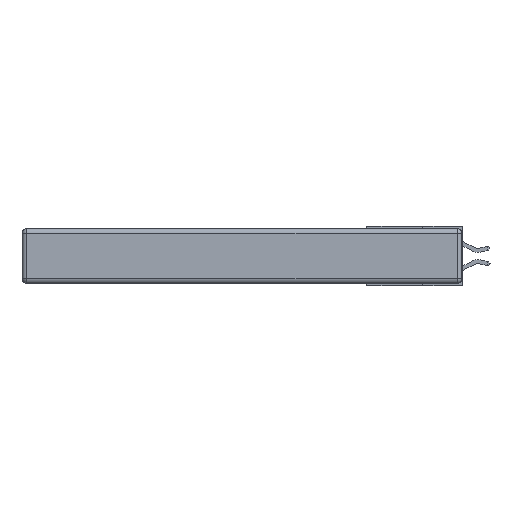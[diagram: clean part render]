
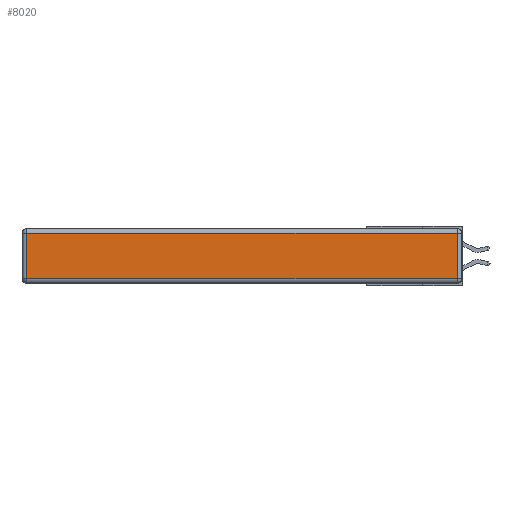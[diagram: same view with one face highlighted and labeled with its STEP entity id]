
A CAD part, left-side view. The second image highlights one B-rep face of the part: STEP entity #8020.
In plain terms, the highlighted planar face has unit normal (-1, 0, 0).
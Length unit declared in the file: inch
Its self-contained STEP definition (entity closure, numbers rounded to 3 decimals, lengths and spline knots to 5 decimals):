
#889 = LINE ( 'NONE', #14037, #1727 ) ;
#997 = CARTESIAN_POINT ( 'NONE',  ( 0., 2.72, -0.03 ) ) ;
#1402 = EDGE_CURVE ( 'NONE', #5670, #11887, #889, .T. ) ;
#1727 = VECTOR ( 'NONE', #5979, 39.37008 ) ;
#2319 = FACE_OUTER_BOUND ( 'NONE', #15746, .T. ) ;
#2559 = CARTESIAN_POINT ( 'NONE',  ( 0., 0., -0.313 ) ) ;
#3452 = DIRECTION ( 'NONE',  ( 0., 0., 1. ) ) ;
#3626 = PLANE ( 'NONE',  #10533 ) ;
#3852 = CARTESIAN_POINT ( 'NONE',  ( 0., 0.03, -0.03 ) ) ;
#4897 = EDGE_CURVE ( 'NONE', #12604, #5670, #10067, .T. ) ;
#5346 = LINE ( 'NONE', #2559, #16307 ) ;
#5541 = CARTESIAN_POINT ( 'NONE',  ( 0., 2.75, -0.03 ) ) ;
#5670 = VERTEX_POINT ( 'NONE', #997 ) ;
#5979 = DIRECTION ( 'NONE',  ( 0., 0., -1. ) ) ;
#6487 = VECTOR ( 'NONE', #8347, 39.37008 ) ;
#6888 = EDGE_CURVE ( 'NONE', #11887, #7565, #5346, .T. ) ;
#7342 = ORIENTED_EDGE ( 'NONE', *, *, #1402, .T. ) ;
#7519 = DIRECTION ( 'NONE',  ( -1., 0., 0. ) ) ;
#7565 = VERTEX_POINT ( 'NONE', #11246 ) ;
#8020 = ADVANCED_FACE ( 'NONE', ( #2319 ), #3626, .T. ) ;
#8347 = DIRECTION ( 'NONE',  ( 0., 1., 0. ) ) ;
#8655 = ORIENTED_EDGE ( 'NONE', *, *, #9060, .T. ) ;
#9060 = EDGE_CURVE ( 'NONE', #7565, #12604, #17295, .T. ) ;
#9147 = DIRECTION ( 'NONE',  ( 0., 0., 1. ) ) ;
#10067 = LINE ( 'NONE', #5541, #6487 ) ;
#10384 = ORIENTED_EDGE ( 'NONE', *, *, #6888, .T. ) ;
#10533 = AXIS2_PLACEMENT_3D ( 'NONE', #11686, #7519, #3452 ) ;
#10699 = CARTESIAN_POINT ( 'NONE',  ( 0., 2.72, -0.313 ) ) ;
#11246 = CARTESIAN_POINT ( 'NONE',  ( 0., 0.03, -0.313 ) ) ;
#11686 = CARTESIAN_POINT ( 'NONE',  ( 0., 0., -0.343 ) ) ;
#11887 = VERTEX_POINT ( 'NONE', #10699 ) ;
#12604 = VERTEX_POINT ( 'NONE', #3852 ) ;
#12836 = ORIENTED_EDGE ( 'NONE', *, *, #4897, .T. ) ;
#13485 = DIRECTION ( 'NONE',  ( 0., -1., 0. ) ) ;
#14037 = CARTESIAN_POINT ( 'NONE',  ( 0., 2.72, -0.343 ) ) ;
#15746 = EDGE_LOOP ( 'NONE', ( #10384, #8655, #12836, #7342 ) ) ;
#15836 = VECTOR ( 'NONE', #9147, 39.37008 ) ;
#16072 = CARTESIAN_POINT ( 'NONE',  ( 0., 0.03, -0.343 ) ) ;
#16307 = VECTOR ( 'NONE', #13485, 39.37008 ) ;
#17295 = LINE ( 'NONE', #16072, #15836 ) ;
